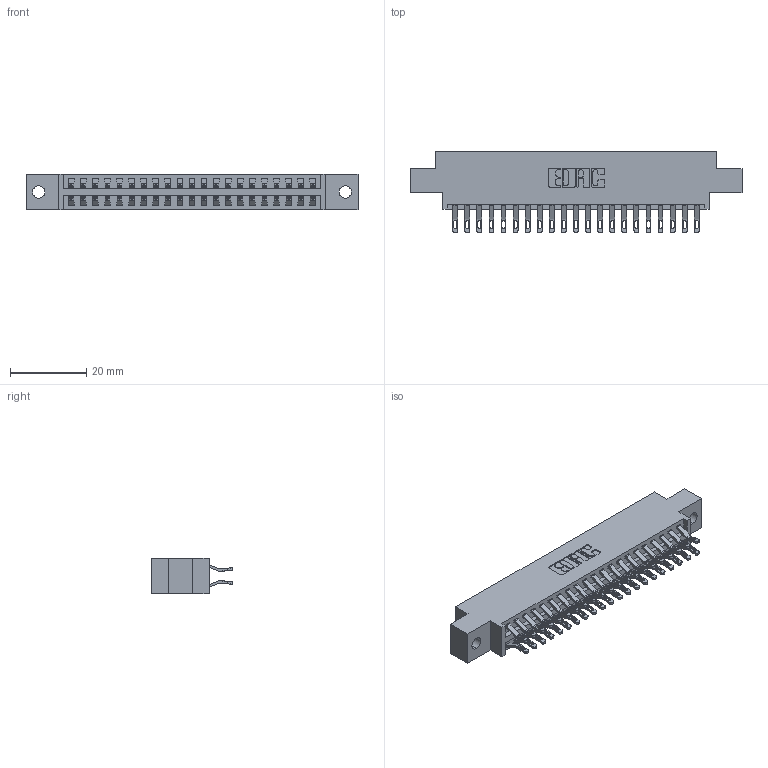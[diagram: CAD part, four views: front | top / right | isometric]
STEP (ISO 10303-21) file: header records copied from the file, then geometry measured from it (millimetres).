
FILE_DESCRIPTION (( 'STEP AP203' ), '1' );
FILE_NAME ('346-042-555-802.STEP', '2022-05-20T04:57:56', ( '' ), ( '' ), 'SwSTEP 2.0', 'SolidWorks 2020', '' );
FILE_SCHEMA (( 'CONFIG_CONTROL_DESIGN' ));
Length unit declared in the file: inch
Products named in the file (3): 345-292-001_555 Tail; 346-042-555-802; 346 Part_0.170 Offset - 0.128 Dia
Assembly tree (43 placements, depth 2):
  346-042-555-802
    346 Part_0.170 Offset - 0.128 Dia
    345-292-001_555 Tail  x42
Bounding box: 87.25 x 21.46 x 9.4 mm (x, y, z)
Volume: 8275.3 mm3; surface area: 11389.5 mm2
Topology: 43 solids, 43 shells, 2562 faces, 8027 edges, 5350 vertices
Faces by surface type: plane 1466, cylinder 1096
Entity records: 16993 total; most frequent: CARTESIAN_POINT 2866, ORIENTED_EDGE 2770, DIRECTION 2545, EDGE_CURVE 1385, VECTOR 1149, LINE 1149, VERTEX_POINT 922, AXIS2_PLACEMENT_3D 698
